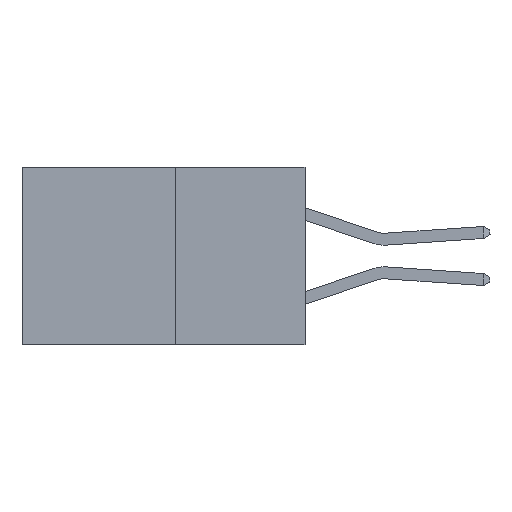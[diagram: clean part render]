
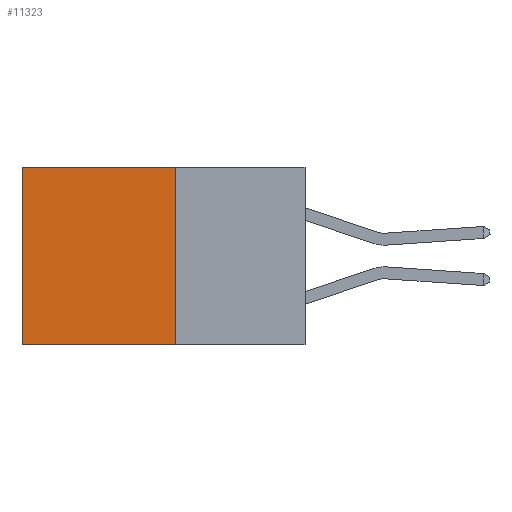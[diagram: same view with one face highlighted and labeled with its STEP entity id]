
A CAD part, left-side view. The second image highlights one B-rep face of the part: STEP entity #11323.
In plain terms, the highlighted planar face has unit normal (-1, 0, 0).
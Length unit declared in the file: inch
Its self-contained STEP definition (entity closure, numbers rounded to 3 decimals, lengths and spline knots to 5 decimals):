
#1420 = PLANE ( 'NONE',  #4855 ) ;
#1443 = CARTESIAN_POINT ( 'NONE',  ( 0.277, 0.59, 0. ) ) ;
#1459 = ORIENTED_EDGE ( 'NONE', *, *, #4626, .T. ) ;
#3066 = CARTESIAN_POINT ( 'NONE',  ( 0.277, 0.27, 0. ) ) ;
#3131 = CARTESIAN_POINT ( 'NONE',  ( 0.277, 0.27, 0. ) ) ;
#3611 = DIRECTION ( 'NONE',  ( 0., 0., -1. ) ) ;
#4159 = VERTEX_POINT ( 'NONE', #1443 ) ;
#4626 = EDGE_CURVE ( 'NONE', #7954, #4159, #10089, .T. ) ;
#4855 = AXIS2_PLACEMENT_3D ( 'NONE', #8769, #9727, #3611 ) ;
#4919 = DIRECTION ( 'NONE',  ( 0., 1., 0. ) ) ;
#5292 = CARTESIAN_POINT ( 'NONE',  ( 0.277, 0.59, -0.37 ) ) ;
#5838 = VECTOR ( 'NONE', #8810, 39.37008 ) ;
#5915 = EDGE_CURVE ( 'NONE', #11599, #6046, #9613, .T. ) ;
#6046 = VERTEX_POINT ( 'NONE', #12936 ) ;
#6889 = CARTESIAN_POINT ( 'NONE',  ( 0.277, 0.27, -0.37 ) ) ;
#6933 = EDGE_LOOP ( 'NONE', ( #9150, #11741, #12037, #1459 ) ) ;
#7565 = VECTOR ( 'NONE', #4919, 39.37008 ) ;
#7652 = EDGE_CURVE ( 'NONE', #7954, #11599, #10771, .T. ) ;
#7954 = VERTEX_POINT ( 'NONE', #3066 ) ;
#8079 = CARTESIAN_POINT ( 'NONE',  ( 0.277, 0.27, -0.37 ) ) ;
#8426 = FACE_OUTER_BOUND ( 'NONE', #6933, .T. ) ;
#8769 = CARTESIAN_POINT ( 'NONE',  ( 0.277, 0.27, -0.37 ) ) ;
#8810 = DIRECTION ( 'NONE',  ( 0., 0., -1. ) ) ;
#8893 = CARTESIAN_POINT ( 'NONE',  ( 0.277, 0.27, -0.37 ) ) ;
#9150 = ORIENTED_EDGE ( 'NONE', *, *, #11835, .T. ) ;
#9613 = LINE ( 'NONE', #8893, #12219 ) ;
#9727 = DIRECTION ( 'NONE',  ( 1., 0., 0. ) ) ;
#10052 = VECTOR ( 'NONE', #13201, 39.37008 ) ;
#10089 = LINE ( 'NONE', #3131, #7565 ) ;
#10771 = LINE ( 'NONE', #6889, #5838 ) ;
#11323 = ADVANCED_FACE ( 'NONE', ( #8426 ), #1420, .F. ) ;
#11599 = VERTEX_POINT ( 'NONE', #8079 ) ;
#11741 = ORIENTED_EDGE ( 'NONE', *, *, #5915, .F. ) ;
#11835 = EDGE_CURVE ( 'NONE', #4159, #6046, #12670, .T. ) ;
#12037 = ORIENTED_EDGE ( 'NONE', *, *, #7652, .F. ) ;
#12219 = VECTOR ( 'NONE', #12725, 39.37008 ) ;
#12670 = LINE ( 'NONE', #5292, #10052 ) ;
#12725 = DIRECTION ( 'NONE',  ( 0., 1., 0. ) ) ;
#12936 = CARTESIAN_POINT ( 'NONE',  ( 0.277, 0.59, -0.37 ) ) ;
#13201 = DIRECTION ( 'NONE',  ( 0., 0., -1. ) ) ;
